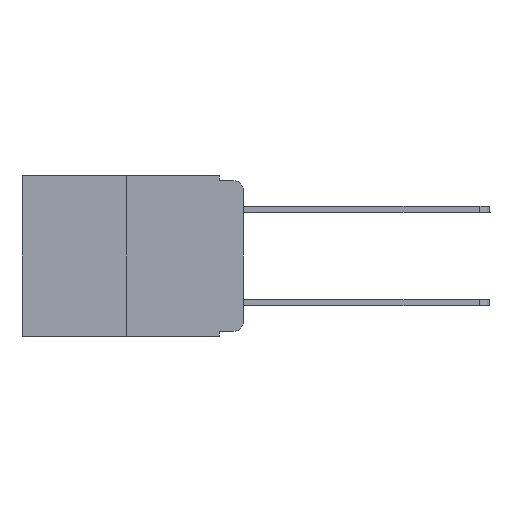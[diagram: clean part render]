
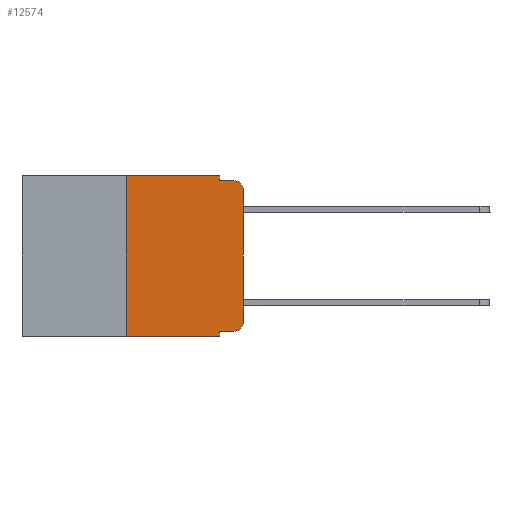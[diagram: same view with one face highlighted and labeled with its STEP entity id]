
A CAD part, left-side view. The second image highlights one B-rep face of the part: STEP entity #12574.
In plain terms, the highlighted planar face has unit normal (-1, 0, 0).
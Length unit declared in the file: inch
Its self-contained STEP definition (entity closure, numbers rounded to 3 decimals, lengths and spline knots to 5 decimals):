
#60 = LINE ( 'NONE', #9783, #13411 ) ;
#208 = LINE ( 'NONE', #1047, #1794 ) ;
#576 = ORIENTED_EDGE ( 'NONE', *, *, #4807, .F. ) ;
#728 = VERTEX_POINT ( 'NONE', #3583 ) ;
#950 = CARTESIAN_POINT ( 'NONE',  ( 0., 0.051, 0. ) ) ;
#960 = ORIENTED_EDGE ( 'NONE', *, *, #12464, .F. ) ;
#1047 = CARTESIAN_POINT ( 'NONE',  ( 0., 0.473, 0. ) ) ;
#1277 = AXIS2_PLACEMENT_3D ( 'NONE', #12504, #5678, #3559 ) ;
#1381 = ORIENTED_EDGE ( 'NONE', *, *, #2447, .F. ) ;
#1794 = VECTOR ( 'NONE', #4498, 39.37008 ) ;
#1988 = EDGE_CURVE ( 'NONE', #2673, #728, #7946, .T. ) ;
#2069 = DIRECTION ( 'NONE',  ( 0., -1., 0. ) ) ;
#2404 = VECTOR ( 'NONE', #9869, 39.37008 ) ;
#2447 = EDGE_CURVE ( 'NONE', #5414, #12053, #4117, .T. ) ;
#2620 = VERTEX_POINT ( 'NONE', #2712 ) ;
#2673 = VERTEX_POINT ( 'NONE', #3163 ) ;
#2712 = CARTESIAN_POINT ( 'NONE',  ( 0., 0.25, -0.343 ) ) ;
#2726 = VERTEX_POINT ( 'NONE', #6285 ) ;
#2764 = CARTESIAN_POINT ( 'NONE',  ( 0., 0.25, 0. ) ) ;
#3112 = VECTOR ( 'NONE', #6090, 39.37008 ) ;
#3163 = CARTESIAN_POINT ( 'NONE',  ( 0., 0., -0.313 ) ) ;
#3380 = DIRECTION ( 'NONE',  ( 0., -1., 0. ) ) ;
#3559 = DIRECTION ( 'NONE',  ( 0., 0., -1. ) ) ;
#3583 = CARTESIAN_POINT ( 'NONE',  ( 0., 0., -0.03 ) ) ;
#3789 = VERTEX_POINT ( 'NONE', #10218 ) ;
#3962 = ORIENTED_EDGE ( 'NONE', *, *, #12644, .T. ) ;
#4117 = LINE ( 'NONE', #950, #11936 ) ;
#4213 = VERTEX_POINT ( 'NONE', #9887 ) ;
#4366 = DIRECTION ( 'NONE',  ( 0., -1., 0. ) ) ;
#4416 = DIRECTION ( 'NONE',  ( 1., 0., 0. ) ) ;
#4498 = DIRECTION ( 'NONE',  ( 0., -1., 0. ) ) ;
#4571 = VECTOR ( 'NONE', #3380, 39.37008 ) ;
#4694 = ORIENTED_EDGE ( 'NONE', *, *, #6696, .F. ) ;
#4715 = ORIENTED_EDGE ( 'NONE', *, *, #8610, .T. ) ;
#4807 = EDGE_CURVE ( 'NONE', #12053, #2726, #60, .T. ) ;
#4877 = EDGE_LOOP ( 'NONE', ( #12638, #3962, #576, #1381, #6769, #4694, #9955, #960, #4715, #14083 ) ) ;
#5378 = AXIS2_PLACEMENT_3D ( 'NONE', #11171, #4416, #8871 ) ;
#5414 = VERTEX_POINT ( 'NONE', #8995 ) ;
#5489 = CARTESIAN_POINT ( 'NONE',  ( 0., 0.051, -0.343 ) ) ;
#5678 = DIRECTION ( 'NONE',  ( -1., 0., 0. ) ) ;
#6090 = DIRECTION ( 'NONE',  ( 0., 0., 1. ) ) ;
#6285 = CARTESIAN_POINT ( 'NONE',  ( 0., 0.02, -0.01 ) ) ;
#6376 = VECTOR ( 'NONE', #14102, 39.37008 ) ;
#6661 = CIRCLE ( 'NONE', #13223, 0.02 ) ;
#6696 = EDGE_CURVE ( 'NONE', #2620, #3789, #7053, .T. ) ;
#6716 = LINE ( 'NONE', #9836, #9013 ) ;
#6769 = ORIENTED_EDGE ( 'NONE', *, *, #13326, .F. ) ;
#7053 = LINE ( 'NONE', #2764, #3112 ) ;
#7192 = DIRECTION ( 'NONE',  ( 0., 0., -1. ) ) ;
#7613 = CARTESIAN_POINT ( 'NONE',  ( 0., 0., 0. ) ) ;
#7622 = CARTESIAN_POINT ( 'NONE',  ( 0., 0.051, -0.333 ) ) ;
#7700 = LINE ( 'NONE', #7622, #4571 ) ;
#7946 = LINE ( 'NONE', #7613, #2404 ) ;
#8042 = EDGE_CURVE ( 'NONE', #4213, #2673, #6661, .T. ) ;
#8137 = CIRCLE ( 'NONE', #1277, 0.02 ) ;
#8610 = EDGE_CURVE ( 'NONE', #10949, #4213, #7700, .T. ) ;
#8645 = VERTEX_POINT ( 'NONE', #5489 ) ;
#8766 = DIRECTION ( 'NONE',  ( 0., 0., -1. ) ) ;
#8871 = DIRECTION ( 'NONE',  ( 0., 0., -1. ) ) ;
#8995 = CARTESIAN_POINT ( 'NONE',  ( 0., 0.051, 0. ) ) ;
#9013 = VECTOR ( 'NONE', #2069, 39.37008 ) ;
#9464 = CARTESIAN_POINT ( 'NONE',  ( 0., 0.02, -0.313 ) ) ;
#9783 = CARTESIAN_POINT ( 'NONE',  ( 0., 0.051, -0.01 ) ) ;
#9836 = CARTESIAN_POINT ( 'NONE',  ( 0., 0.473, -0.343 ) ) ;
#9869 = DIRECTION ( 'NONE',  ( 0., 0., 1. ) ) ;
#9887 = CARTESIAN_POINT ( 'NONE',  ( 0., 0.02, -0.333 ) ) ;
#9955 = ORIENTED_EDGE ( 'NONE', *, *, #12431, .T. ) ;
#10218 = CARTESIAN_POINT ( 'NONE',  ( 0., 0.25, 0. ) ) ;
#10949 = VERTEX_POINT ( 'NONE', #12017 ) ;
#11171 = CARTESIAN_POINT ( 'NONE',  ( 0., 0.473, 0. ) ) ;
#11587 = FACE_OUTER_BOUND ( 'NONE', #4877, .T. ) ;
#11631 = DIRECTION ( 'NONE',  ( -1., 0., 0. ) ) ;
#11936 = VECTOR ( 'NONE', #8766, 39.37008 ) ;
#11957 = LINE ( 'NONE', #11961, #6376 ) ;
#11961 = CARTESIAN_POINT ( 'NONE',  ( 0., 0.051, 0. ) ) ;
#12017 = CARTESIAN_POINT ( 'NONE',  ( 0., 0.051, -0.333 ) ) ;
#12053 = VERTEX_POINT ( 'NONE', #12419 ) ;
#12229 = PLANE ( 'NONE',  #5378 ) ;
#12419 = CARTESIAN_POINT ( 'NONE',  ( 0., 0.051, -0.01 ) ) ;
#12431 = EDGE_CURVE ( 'NONE', #2620, #8645, #6716, .T. ) ;
#12464 = EDGE_CURVE ( 'NONE', #10949, #8645, #11957, .T. ) ;
#12504 = CARTESIAN_POINT ( 'NONE',  ( 0., 0.02, -0.03 ) ) ;
#12574 = ADVANCED_FACE ( 'NONE', ( #11587 ), #12229, .F. ) ;
#12638 = ORIENTED_EDGE ( 'NONE', *, *, #1988, .T. ) ;
#12644 = EDGE_CURVE ( 'NONE', #728, #2726, #8137, .T. ) ;
#13223 = AXIS2_PLACEMENT_3D ( 'NONE', #9464, #11631, #7192 ) ;
#13326 = EDGE_CURVE ( 'NONE', #3789, #5414, #208, .T. ) ;
#13411 = VECTOR ( 'NONE', #4366, 39.37008 ) ;
#14083 = ORIENTED_EDGE ( 'NONE', *, *, #8042, .T. ) ;
#14102 = DIRECTION ( 'NONE',  ( 0., 0., -1. ) ) ;
